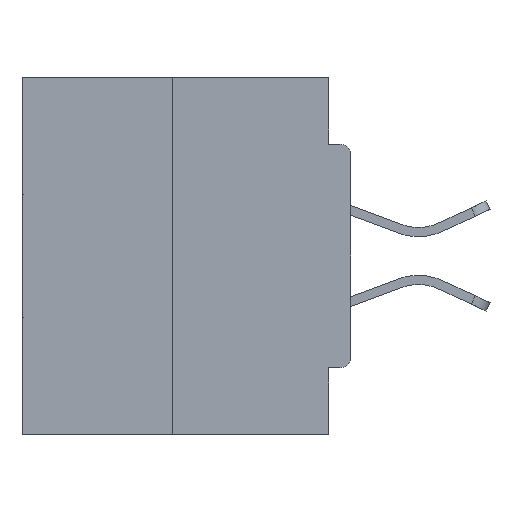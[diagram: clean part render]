
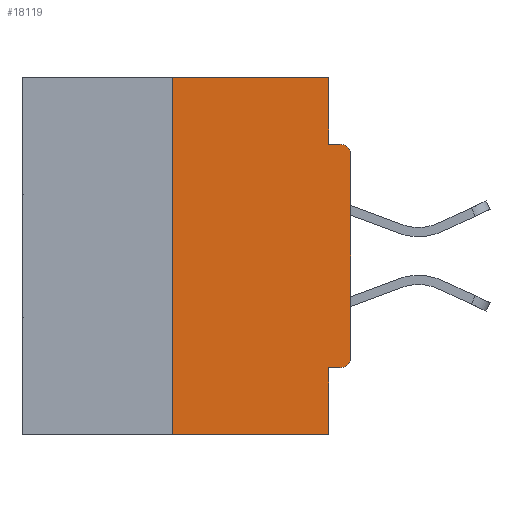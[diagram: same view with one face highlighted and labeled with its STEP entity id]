
A CAD part, left-side view. The second image highlights one B-rep face of the part: STEP entity #18119.
In plain terms, the highlighted planar face has unit normal (-1, 0, 0).
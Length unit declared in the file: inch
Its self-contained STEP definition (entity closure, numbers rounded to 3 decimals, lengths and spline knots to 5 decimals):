
#252 = EDGE_CURVE ( 'NONE', #9128, #1221, #22264, .T. ) ;
#562 = CARTESIAN_POINT ( 'NONE',  ( 0., 0.46, 0. ) ) ;
#776 = LINE ( 'NONE', #9934, #38339 ) ;
#785 = VERTEX_POINT ( 'NONE', #22893 ) ;
#862 = ORIENTED_EDGE ( 'NONE', *, *, #10663, .F. ) ;
#1221 = VERTEX_POINT ( 'NONE', #26306 ) ;
#1944 = VERTEX_POINT ( 'NONE', #35078 ) ;
#2817 = DIRECTION ( 'NONE',  ( 0., 0., -1. ) ) ;
#3343 = VERTEX_POINT ( 'NONE', #13523 ) ;
#3763 = AXIS2_PLACEMENT_3D ( 'NONE', #35549, #18217, #30256 ) ;
#3899 = CARTESIAN_POINT ( 'NONE',  ( 0., 0.031, -0.5 ) ) ;
#4049 = EDGE_CURVE ( 'NONE', #785, #3343, #17760, .T. ) ;
#4383 = DIRECTION ( 'NONE',  ( 0., 0., 1. ) ) ;
#4507 = LINE ( 'NONE', #16736, #34184 ) ;
#5204 = EDGE_LOOP ( 'NONE', ( #38340, #23870, #7246, #26465, #862, #5333, #10978, #19365, #16114, #23060 ) ) ;
#5333 = ORIENTED_EDGE ( 'NONE', *, *, #252, .T. ) ;
#6300 = DIRECTION ( 'NONE',  ( 0., 0., -1. ) ) ;
#7246 = ORIENTED_EDGE ( 'NONE', *, *, #29352, .T. ) ;
#7688 = VECTOR ( 'NONE', #36853, 39.37008 ) ;
#7916 = DIRECTION ( 'NONE',  ( 0., 0., 1. ) ) ;
#7974 = LINE ( 'NONE', #23779, #18666 ) ;
#8727 = EDGE_CURVE ( 'NONE', #27518, #12932, #19531, .T. ) ;
#8949 = VECTOR ( 'NONE', #16603, 39.37008 ) ;
#9128 = VERTEX_POINT ( 'NONE', #10521 ) ;
#9853 = DIRECTION ( 'NONE',  ( 0., 0., -1. ) ) ;
#9934 = CARTESIAN_POINT ( 'NONE',  ( 0., 0., -0.4065 ) ) ;
#10463 = FACE_OUTER_BOUND ( 'NONE', #5204, .T. ) ;
#10521 = CARTESIAN_POINT ( 'NONE',  ( 0., 0.015, -0.4065 ) ) ;
#10635 = CARTESIAN_POINT ( 'NONE',  ( 0., 0., -0.0935 ) ) ;
#10653 = VECTOR ( 'NONE', #4383, 39.37008 ) ;
#10663 = EDGE_CURVE ( 'NONE', #9128, #27518, #776, .T. ) ;
#10978 = ORIENTED_EDGE ( 'NONE', *, *, #27410, .T. ) ;
#11689 = DIRECTION ( 'NONE',  ( 0., -1., 0. ) ) ;
#12932 = VERTEX_POINT ( 'NONE', #36622 ) ;
#13167 = CARTESIAN_POINT ( 'NONE',  ( 0., 0.031, 0. ) ) ;
#13523 = CARTESIAN_POINT ( 'NONE',  ( 0., 0.015, -0.0935 ) ) ;
#14386 = VECTOR ( 'NONE', #9853, 39.37008 ) ;
#16114 = ORIENTED_EDGE ( 'NONE', *, *, #4049, .F. ) ;
#16603 = DIRECTION ( 'NONE',  ( 0., -1., 0. ) ) ;
#16736 = CARTESIAN_POINT ( 'NONE',  ( 0., 0.25, 0. ) ) ;
#17760 = LINE ( 'NONE', #10635, #8949 ) ;
#17972 = DIRECTION ( 'NONE',  ( -1., 0., 0. ) ) ;
#18119 = ADVANCED_FACE ( 'NONE', ( #10463 ), #28367, .F. ) ;
#18217 = DIRECTION ( 'NONE',  ( -1., 0., 0. ) ) ;
#18666 = VECTOR ( 'NONE', #6300, 39.37008 ) ;
#19321 = LINE ( 'NONE', #562, #7688 ) ;
#19365 = ORIENTED_EDGE ( 'NONE', *, *, #30074, .T. ) ;
#19531 = LINE ( 'NONE', #3899, #14386 ) ;
#19733 = DIRECTION ( 'NONE',  ( 1., 0., 0. ) ) ;
#19988 = DIRECTION ( 'NONE',  ( 0., 0., -1. ) ) ;
#21915 = CARTESIAN_POINT ( 'NONE',  ( 0., 0.25, 0. ) ) ;
#22264 = CIRCLE ( 'NONE', #3763, 0.015 ) ;
#22893 = CARTESIAN_POINT ( 'NONE',  ( 0., 0.031, -0.0935 ) ) ;
#23060 = ORIENTED_EDGE ( 'NONE', *, *, #30543, .F. ) ;
#23413 = EDGE_CURVE ( 'NONE', #28255, #37019, #4507, .T. ) ;
#23555 = CARTESIAN_POINT ( 'NONE',  ( 0., 0.015, -0.1085 ) ) ;
#23779 = CARTESIAN_POINT ( 'NONE',  ( 0., 0.031, 0. ) ) ;
#23870 = ORIENTED_EDGE ( 'NONE', *, *, #23413, .F. ) ;
#23972 = VECTOR ( 'NONE', #11689, 39.37008 ) ;
#24756 = CARTESIAN_POINT ( 'NONE',  ( 0., 0.031, -0.4065 ) ) ;
#26306 = CARTESIAN_POINT ( 'NONE',  ( 0., 0., -0.3915 ) ) ;
#26465 = ORIENTED_EDGE ( 'NONE', *, *, #8727, .F. ) ;
#26522 = AXIS2_PLACEMENT_3D ( 'NONE', #23555, #17972, #2817 ) ;
#26663 = CIRCLE ( 'NONE', #26522, 0.015 ) ;
#27410 = EDGE_CURVE ( 'NONE', #1221, #1944, #35262, .T. ) ;
#27518 = VERTEX_POINT ( 'NONE', #24756 ) ;
#28255 = VERTEX_POINT ( 'NONE', #29809 ) ;
#28367 = PLANE ( 'NONE',  #33004 ) ;
#29209 = EDGE_CURVE ( 'NONE', #37019, #34396, #19321, .T. ) ;
#29312 = CARTESIAN_POINT ( 'NONE',  ( 0., 0.46, -0.5 ) ) ;
#29352 = EDGE_CURVE ( 'NONE', #28255, #12932, #37844, .T. ) ;
#29809 = CARTESIAN_POINT ( 'NONE',  ( 0., 0.25, -0.5 ) ) ;
#30074 = EDGE_CURVE ( 'NONE', #1944, #3343, #26663, .T. ) ;
#30256 = DIRECTION ( 'NONE',  ( 0., 0., -1. ) ) ;
#30543 = EDGE_CURVE ( 'NONE', #34396, #785, #7974, .T. ) ;
#33004 = AXIS2_PLACEMENT_3D ( 'NONE', #37700, #19733, #19988 ) ;
#33397 = DIRECTION ( 'NONE',  ( 0., 1., 0. ) ) ;
#34184 = VECTOR ( 'NONE', #7916, 39.37008 ) ;
#34396 = VERTEX_POINT ( 'NONE', #13167 ) ;
#34569 = CARTESIAN_POINT ( 'NONE',  ( 0., 0., 0. ) ) ;
#35078 = CARTESIAN_POINT ( 'NONE',  ( 0., 0., -0.1085 ) ) ;
#35262 = LINE ( 'NONE', #34569, #10653 ) ;
#35549 = CARTESIAN_POINT ( 'NONE',  ( 0., 0.015, -0.3915 ) ) ;
#36622 = CARTESIAN_POINT ( 'NONE',  ( 0., 0.031, -0.5 ) ) ;
#36853 = DIRECTION ( 'NONE',  ( 0., -1., 0. ) ) ;
#37019 = VERTEX_POINT ( 'NONE', #21915 ) ;
#37700 = CARTESIAN_POINT ( 'NONE',  ( 0., 0.46, 0. ) ) ;
#37844 = LINE ( 'NONE', #29312, #23972 ) ;
#38339 = VECTOR ( 'NONE', #33397, 39.37008 ) ;
#38340 = ORIENTED_EDGE ( 'NONE', *, *, #29209, .F. ) ;
